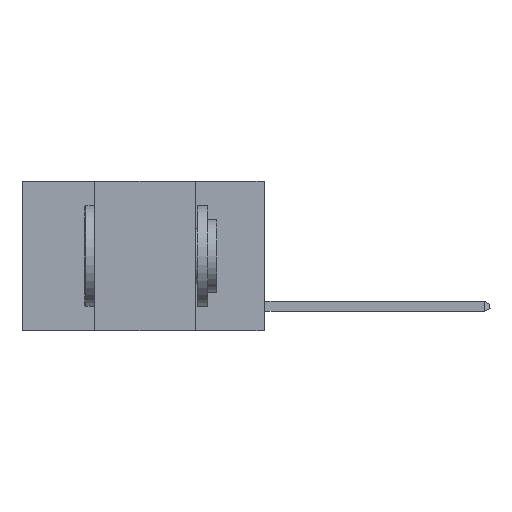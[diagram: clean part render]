
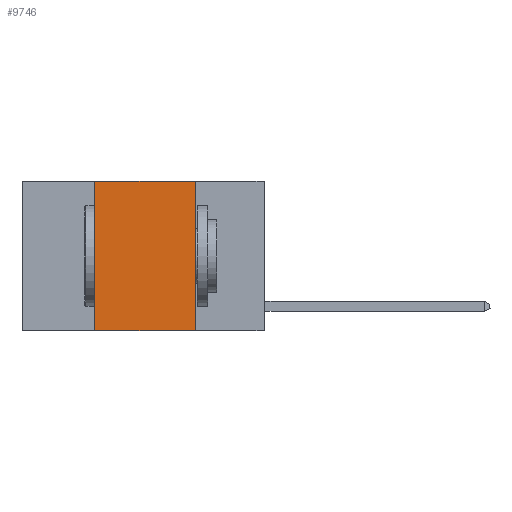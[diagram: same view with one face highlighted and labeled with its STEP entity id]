
A CAD part, left-side view. The second image highlights one B-rep face of the part: STEP entity #9746.
In plain terms, the highlighted planar face has unit normal (-1, 0, 0).
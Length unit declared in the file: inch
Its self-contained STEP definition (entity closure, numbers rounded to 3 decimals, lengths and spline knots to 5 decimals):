
#1187 = DIRECTION ( 'NONE',  ( 0., -1., 0. ) ) ;
#1266 = LINE ( 'NONE', #9899, #12137 ) ;
#1389 = EDGE_CURVE ( 'NONE', #2782, #9261, #6360, .T. ) ;
#1616 = LINE ( 'NONE', #9184, #3430 ) ;
#1708 = DIRECTION ( 'NONE',  ( 1., 0., 0. ) ) ;
#2102 = ORIENTED_EDGE ( 'NONE', *, *, #8959, .F. ) ;
#2231 = DIRECTION ( 'NONE',  ( 0., 0., 1. ) ) ;
#2782 = VERTEX_POINT ( 'NONE', #13144 ) ;
#2979 = ORIENTED_EDGE ( 'NONE', *, *, #4439, .F. ) ;
#3112 = VECTOR ( 'NONE', #3317, 39.37008 ) ;
#3317 = DIRECTION ( 'NONE',  ( 0., -1., 0. ) ) ;
#3430 = VECTOR ( 'NONE', #13590, 39.37008 ) ;
#4327 = ORIENTED_EDGE ( 'NONE', *, *, #11302, .F. ) ;
#4439 = EDGE_CURVE ( 'NONE', #8220, #9261, #1616, .T. ) ;
#5827 = AXIS2_PLACEMENT_3D ( 'NONE', #11517, #1708, #8342 ) ;
#6360 = LINE ( 'NONE', #13141, #6761 ) ;
#6761 = VECTOR ( 'NONE', #1187, 39.37008 ) ;
#7384 = PLANE ( 'NONE',  #5827 ) ;
#8220 = VERTEX_POINT ( 'NONE', #13322 ) ;
#8342 = DIRECTION ( 'NONE',  ( 0., 0., -1. ) ) ;
#8400 = VERTEX_POINT ( 'NONE', #12947 ) ;
#8489 = FACE_OUTER_BOUND ( 'NONE', #12771, .T. ) ;
#8959 = EDGE_CURVE ( 'NONE', #8400, #8220, #13133, .T. ) ;
#9184 = CARTESIAN_POINT ( 'NONE',  ( 0., 0.17, 0. ) ) ;
#9261 = VERTEX_POINT ( 'NONE', #10581 ) ;
#9746 = ADVANCED_FACE ( 'NONE', ( #8489 ), #7384, .F. ) ;
#9885 = CARTESIAN_POINT ( 'NONE',  ( 0., 0.6, 0. ) ) ;
#9899 = CARTESIAN_POINT ( 'NONE',  ( 0., 0.42, 0. ) ) ;
#10581 = CARTESIAN_POINT ( 'NONE',  ( 0., 0.17, -0.37 ) ) ;
#11302 = EDGE_CURVE ( 'NONE', #2782, #8400, #1266, .T. ) ;
#11517 = CARTESIAN_POINT ( 'NONE',  ( 0., 0.6, 0. ) ) ;
#11783 = ORIENTED_EDGE ( 'NONE', *, *, #1389, .T. ) ;
#12137 = VECTOR ( 'NONE', #2231, 39.37008 ) ;
#12771 = EDGE_LOOP ( 'NONE', ( #2979, #2102, #4327, #11783 ) ) ;
#12947 = CARTESIAN_POINT ( 'NONE',  ( 0., 0.42, 0. ) ) ;
#13133 = LINE ( 'NONE', #9885, #3112 ) ;
#13141 = CARTESIAN_POINT ( 'NONE',  ( 0., 0.6, -0.37 ) ) ;
#13144 = CARTESIAN_POINT ( 'NONE',  ( 0., 0.42, -0.37 ) ) ;
#13322 = CARTESIAN_POINT ( 'NONE',  ( 0., 0.17, 0. ) ) ;
#13590 = DIRECTION ( 'NONE',  ( 0., 0., -1. ) ) ;
